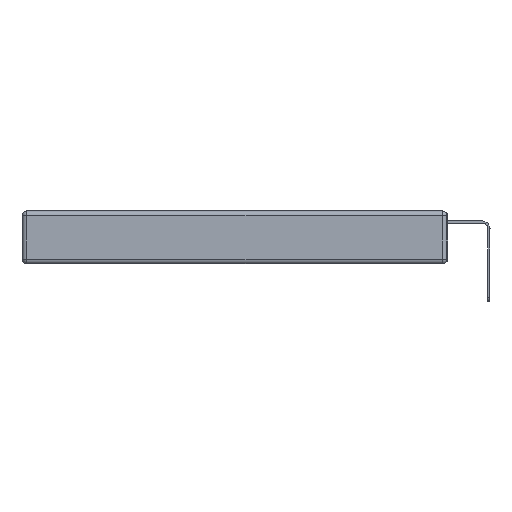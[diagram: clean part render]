
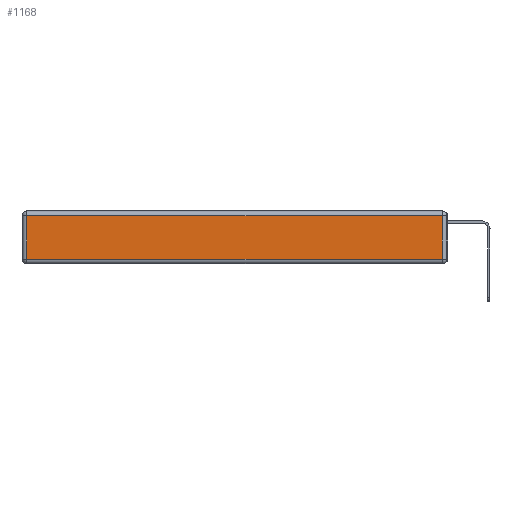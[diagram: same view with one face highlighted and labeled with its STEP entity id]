
A CAD part, left-side view. The second image highlights one B-rep face of the part: STEP entity #1168.
In plain terms, the highlighted planar face has unit normal (-1, 0, 0).
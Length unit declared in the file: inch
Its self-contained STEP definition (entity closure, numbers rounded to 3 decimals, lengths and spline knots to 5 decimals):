
#1168 = ADVANCED_FACE ( 'NONE', ( #21804 ), #3809, .T. ) ;
#2226 = ORIENTED_EDGE ( 'NONE', *, *, #14990, .T. ) ;
#2313 = VERTEX_POINT ( 'NONE', #12555 ) ;
#2502 = ORIENTED_EDGE ( 'NONE', *, *, #11862, .T. ) ;
#3809 = PLANE ( 'NONE',  #8944 ) ;
#4339 = VERTEX_POINT ( 'NONE', #14810 ) ;
#5270 = VECTOR ( 'NONE', #13479, 39.37008 ) ;
#5521 = DIRECTION ( 'NONE',  ( 0., -1., 0. ) ) ;
#5786 = CARTESIAN_POINT ( 'NONE',  ( 0., 0., -0.343 ) ) ;
#6344 = CARTESIAN_POINT ( 'NONE',  ( 0., 2.75, -0.03 ) ) ;
#8124 = EDGE_LOOP ( 'NONE', ( #11468, #2226, #17280, #2502 ) ) ;
#8528 = VERTEX_POINT ( 'NONE', #13505 ) ;
#8719 = VECTOR ( 'NONE', #12015, 39.37008 ) ;
#8944 = AXIS2_PLACEMENT_3D ( 'NONE', #5786, #11057, #9292 ) ;
#9144 = LINE ( 'NONE', #12788, #14680 ) ;
#9292 = DIRECTION ( 'NONE',  ( 0., 0., 1. ) ) ;
#10963 = DIRECTION ( 'NONE',  ( 0., 0., -1. ) ) ;
#11057 = DIRECTION ( 'NONE',  ( -1., 0., 0. ) ) ;
#11468 = ORIENTED_EDGE ( 'NONE', *, *, #16327, .T. ) ;
#11862 = EDGE_CURVE ( 'NONE', #8528, #2313, #22309, .T. ) ;
#12015 = DIRECTION ( 'NONE',  ( 0., 0., 1. ) ) ;
#12555 = CARTESIAN_POINT ( 'NONE',  ( 0., 2.72, -0.313 ) ) ;
#12786 = EDGE_CURVE ( 'NONE', #20461, #8528, #18699, .T. ) ;
#12788 = CARTESIAN_POINT ( 'NONE',  ( 0., 0., -0.313 ) ) ;
#13479 = DIRECTION ( 'NONE',  ( 0., 1., 0. ) ) ;
#13505 = CARTESIAN_POINT ( 'NONE',  ( 0., 2.72, -0.03 ) ) ;
#13948 = LINE ( 'NONE', #15473, #8719 ) ;
#14431 = CARTESIAN_POINT ( 'NONE',  ( 0., 2.72, -0.343 ) ) ;
#14632 = VECTOR ( 'NONE', #10963, 39.37008 ) ;
#14680 = VECTOR ( 'NONE', #5521, 39.37008 ) ;
#14810 = CARTESIAN_POINT ( 'NONE',  ( 0., 0.03, -0.313 ) ) ;
#14990 = EDGE_CURVE ( 'NONE', #4339, #20461, #13948, .T. ) ;
#15473 = CARTESIAN_POINT ( 'NONE',  ( 0., 0.03, -0.343 ) ) ;
#16327 = EDGE_CURVE ( 'NONE', #2313, #4339, #9144, .T. ) ;
#17280 = ORIENTED_EDGE ( 'NONE', *, *, #12786, .T. ) ;
#18495 = CARTESIAN_POINT ( 'NONE',  ( 0., 0.03, -0.03 ) ) ;
#18699 = LINE ( 'NONE', #6344, #5270 ) ;
#20461 = VERTEX_POINT ( 'NONE', #18495 ) ;
#21804 = FACE_OUTER_BOUND ( 'NONE', #8124, .T. ) ;
#22309 = LINE ( 'NONE', #14431, #14632 ) ;
